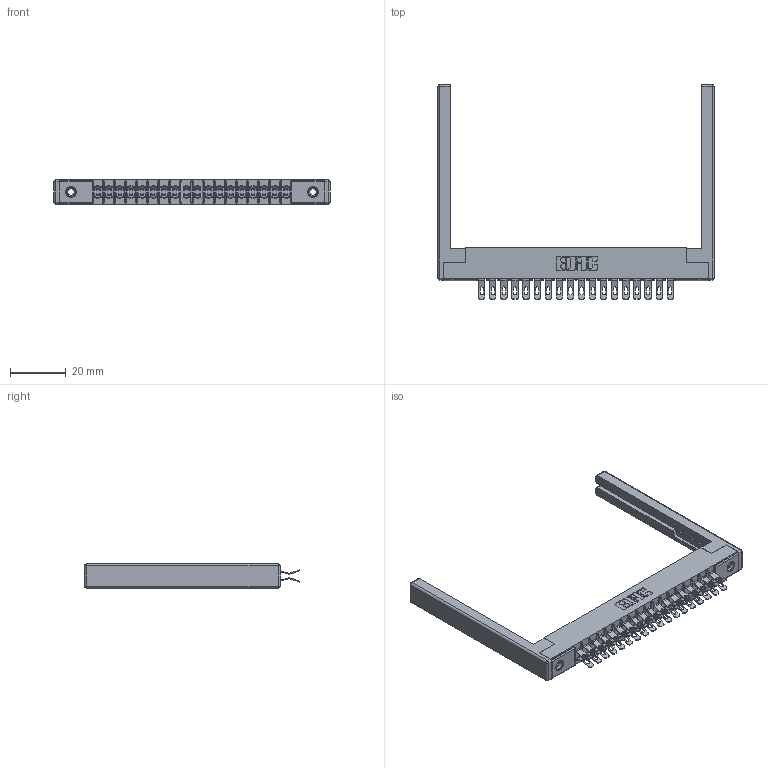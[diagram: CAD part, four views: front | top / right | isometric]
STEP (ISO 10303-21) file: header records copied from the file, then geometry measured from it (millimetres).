
FILE_DESCRIPTION (( 'STEP AP203' ), '1' );
FILE_NAME ('305-036-555-568.STEP', '2019-09-09T18:12:27', ( '' ), ( '' ), 'SwSTEP 2.0', 'SolidWorks 2016', '' );
FILE_SCHEMA (( 'CONFIG_CONTROL_DESIGN' ));
Length unit declared in the file: inch
Products named in the file (5): 345-250-001_345-250-001-102; 307-220-068; 305-290-001_555; 305-036-555-568; 305 Part_.156 Dia
Assembly tree (41 placements, depth 2):
  305-036-555-568
    305 Part_.156 Dia
    305-290-001_555  x36
    345-250-001_345-250-001-102  x2
    307-220-068  x2
Bounding box: 98.76 x 76.71 x 8.71 mm (x, y, z)
Volume: 10625.7 mm3; surface area: 16403.5 mm2
Topology: 41 solids, 41 shells, 2646 faces, 7816 edges, 5092 vertices
Faces by surface type: plane 1308, cylinder 1242, sphere 80, cone 12, torus 4
Entity records: 25794 total; most frequent: CARTESIAN_POINT 4259, ORIENTED_EDGE 4206, DIRECTION 4153, EDGE_CURVE 2103, VECTOR 1645, LINE 1645, VERTEX_POINT 1344, AXIS2_PLACEMENT_3D 1254
